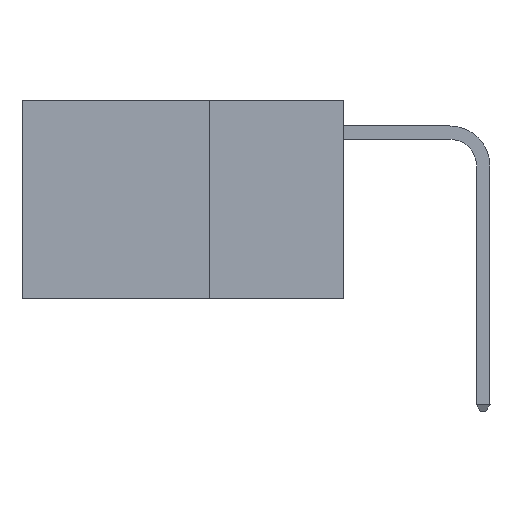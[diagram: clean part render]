
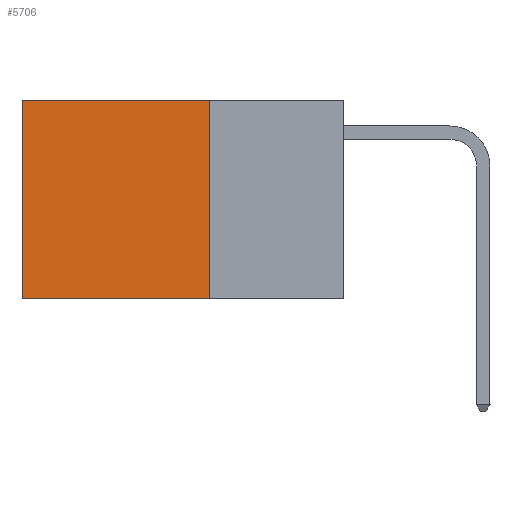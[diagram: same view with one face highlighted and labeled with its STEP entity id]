
A CAD part, left-side view. The second image highlights one B-rep face of the part: STEP entity #5706.
In plain terms, the highlighted planar face has unit normal (-1, 0, 0).
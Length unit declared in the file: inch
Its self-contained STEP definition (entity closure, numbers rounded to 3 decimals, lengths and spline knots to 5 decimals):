
#222 = EDGE_CURVE ( 'NONE', #7244, #5906, #5846, .T. ) ;
#293 = CARTESIAN_POINT ( 'NONE',  ( 0.2625, 0.6, -0.37 ) ) ;
#315 = DIRECTION ( 'NONE',  ( 0., 1., 0. ) ) ;
#316 = AXIS2_PLACEMENT_3D ( 'NONE', #1266, #1253, #1236 ) ;
#1114 = EDGE_LOOP ( 'NONE', ( #9082, #2388, #5249, #2815 ) ) ;
#1236 = DIRECTION ( 'NONE',  ( 0., 0., -1. ) ) ;
#1253 = DIRECTION ( 'NONE',  ( 1., 0., 0. ) ) ;
#1266 = CARTESIAN_POINT ( 'NONE',  ( 0.2625, 0.25, 0. ) ) ;
#1344 = PLANE ( 'NONE',  #316 ) ;
#2217 = LINE ( 'NONE', #3001, #8669 ) ;
#2388 = ORIENTED_EDGE ( 'NONE', *, *, #10355, .F. ) ;
#2452 = CARTESIAN_POINT ( 'NONE',  ( 0.2625, 0.6, 0. ) ) ;
#2815 = ORIENTED_EDGE ( 'NONE', *, *, #7679, .T. ) ;
#2868 = DIRECTION ( 'NONE',  ( 0., 1., 0. ) ) ;
#3001 = CARTESIAN_POINT ( 'NONE',  ( 0.2625, 0.25, -0.37 ) ) ;
#3104 = CARTESIAN_POINT ( 'NONE',  ( 0.2625, 0.25, 0. ) ) ;
#3219 = CARTESIAN_POINT ( 'NONE',  ( 0.2625, 0.25, 0. ) ) ;
#3606 = LINE ( 'NONE', #3104, #7952 ) ;
#4459 = LINE ( 'NONE', #8502, #8801 ) ;
#5249 = ORIENTED_EDGE ( 'NONE', *, *, #10539, .F. ) ;
#5706 = ADVANCED_FACE ( 'NONE', ( #10206 ), #1344, .F. ) ;
#5795 = VECTOR ( 'NONE', #10558, 39.37008 ) ;
#5846 = LINE ( 'NONE', #2452, #5795 ) ;
#5860 = CARTESIAN_POINT ( 'NONE',  ( 0.2625, 0.25, -0.37 ) ) ;
#5906 = VERTEX_POINT ( 'NONE', #293 ) ;
#7051 = CARTESIAN_POINT ( 'NONE',  ( 0.2625, 0.6, 0. ) ) ;
#7244 = VERTEX_POINT ( 'NONE', #7051 ) ;
#7679 = EDGE_CURVE ( 'NONE', #9170, #7244, #3606, .T. ) ;
#7952 = VECTOR ( 'NONE', #2868, 39.37008 ) ;
#8502 = CARTESIAN_POINT ( 'NONE',  ( 0.2625, 0.25, 0. ) ) ;
#8669 = VECTOR ( 'NONE', #315, 39.37008 ) ;
#8801 = VECTOR ( 'NONE', #10264, 39.37008 ) ;
#8914 = VERTEX_POINT ( 'NONE', #5860 ) ;
#9082 = ORIENTED_EDGE ( 'NONE', *, *, #222, .T. ) ;
#9170 = VERTEX_POINT ( 'NONE', #3219 ) ;
#10206 = FACE_OUTER_BOUND ( 'NONE', #1114, .T. ) ;
#10264 = DIRECTION ( 'NONE',  ( 0., 0., -1. ) ) ;
#10355 = EDGE_CURVE ( 'NONE', #8914, #5906, #2217, .T. ) ;
#10539 = EDGE_CURVE ( 'NONE', #9170, #8914, #4459, .T. ) ;
#10558 = DIRECTION ( 'NONE',  ( 0., 0., -1. ) ) ;
